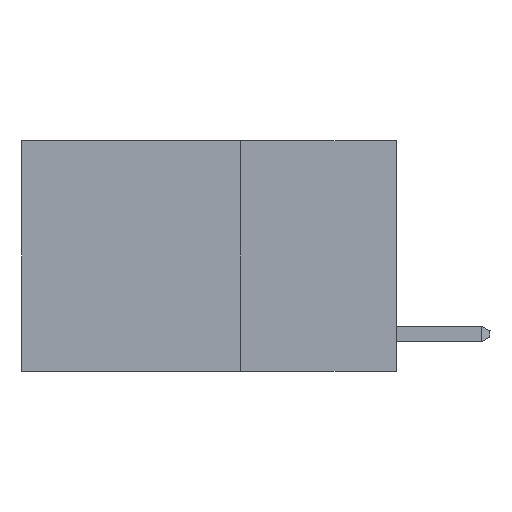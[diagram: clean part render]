
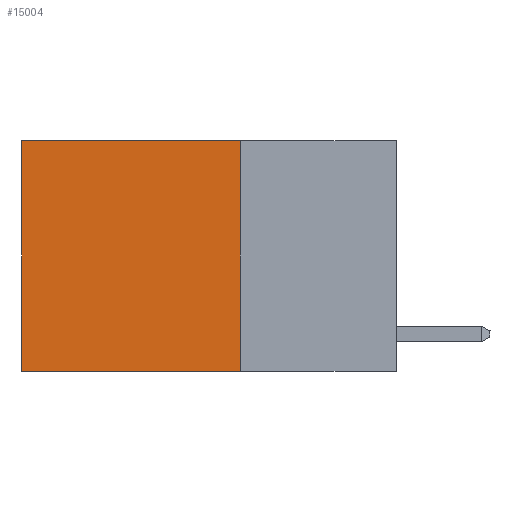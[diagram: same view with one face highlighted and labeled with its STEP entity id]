
A CAD part, left-side view. The second image highlights one B-rep face of the part: STEP entity #15004.
In plain terms, the highlighted planar face has unit normal (-1, 0, 0).
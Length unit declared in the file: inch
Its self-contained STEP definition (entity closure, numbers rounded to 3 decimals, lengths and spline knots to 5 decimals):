
#166 = CARTESIAN_POINT ( 'NONE',  ( 0.2625, 0.25, 0. ) ) ;
#193 = DIRECTION ( 'NONE',  ( 0., 0., -1. ) ) ;
#298 = ORIENTED_EDGE ( 'NONE', *, *, #2915, .T. ) ;
#578 = VECTOR ( 'NONE', #17614, 39.37008 ) ;
#2310 = VERTEX_POINT ( 'NONE', #4918 ) ;
#2915 = EDGE_CURVE ( 'NONE', #11059, #16222, #8805, .T. ) ;
#3116 = EDGE_LOOP ( 'NONE', ( #16686, #7817, #7000, #298 ) ) ;
#4749 = PLANE ( 'NONE',  #6871 ) ;
#4918 = CARTESIAN_POINT ( 'NONE',  ( 0.2625, 0.25, -0.37 ) ) ;
#5275 = DIRECTION ( 'NONE',  ( 0., 0., -1. ) ) ;
#5807 = VECTOR ( 'NONE', #193, 39.37008 ) ;
#6135 = EDGE_CURVE ( 'NONE', #16222, #12119, #17280, .T. ) ;
#6406 = CARTESIAN_POINT ( 'NONE',  ( 0.2625, 0.6, 0. ) ) ;
#6632 = FACE_OUTER_BOUND ( 'NONE', #3116, .T. ) ;
#6871 = AXIS2_PLACEMENT_3D ( 'NONE', #166, #12407, #13979 ) ;
#7000 = ORIENTED_EDGE ( 'NONE', *, *, #13277, .F. ) ;
#7817 = ORIENTED_EDGE ( 'NONE', *, *, #12506, .F. ) ;
#7934 = CARTESIAN_POINT ( 'NONE',  ( 0.2625, 0.25, 0. ) ) ;
#8725 = VECTOR ( 'NONE', #5275, 39.37008 ) ;
#8805 = LINE ( 'NONE', #19239, #578 ) ;
#10283 = VECTOR ( 'NONE', #13025, 39.37008 ) ;
#11059 = VERTEX_POINT ( 'NONE', #12666 ) ;
#12119 = VERTEX_POINT ( 'NONE', #16141 ) ;
#12407 = DIRECTION ( 'NONE',  ( 1., 0., 0. ) ) ;
#12506 = EDGE_CURVE ( 'NONE', #2310, #12119, #14328, .T. ) ;
#12666 = CARTESIAN_POINT ( 'NONE',  ( 0.2625, 0.25, 0. ) ) ;
#13025 = DIRECTION ( 'NONE',  ( 0., 1., 0. ) ) ;
#13277 = EDGE_CURVE ( 'NONE', #11059, #2310, #17873, .T. ) ;
#13973 = CARTESIAN_POINT ( 'NONE',  ( 0.2625, 0.6, 0. ) ) ;
#13979 = DIRECTION ( 'NONE',  ( 0., 0., -1. ) ) ;
#14328 = LINE ( 'NONE', #17374, #10283 ) ;
#15004 = ADVANCED_FACE ( 'NONE', ( #6632 ), #4749, .F. ) ;
#16141 = CARTESIAN_POINT ( 'NONE',  ( 0.2625, 0.6, -0.37 ) ) ;
#16222 = VERTEX_POINT ( 'NONE', #6406 ) ;
#16686 = ORIENTED_EDGE ( 'NONE', *, *, #6135, .T. ) ;
#17280 = LINE ( 'NONE', #13973, #8725 ) ;
#17374 = CARTESIAN_POINT ( 'NONE',  ( 0.2625, 0.25, -0.37 ) ) ;
#17614 = DIRECTION ( 'NONE',  ( 0., 1., 0. ) ) ;
#17873 = LINE ( 'NONE', #7934, #5807 ) ;
#19239 = CARTESIAN_POINT ( 'NONE',  ( 0.2625, 0.25, 0. ) ) ;
